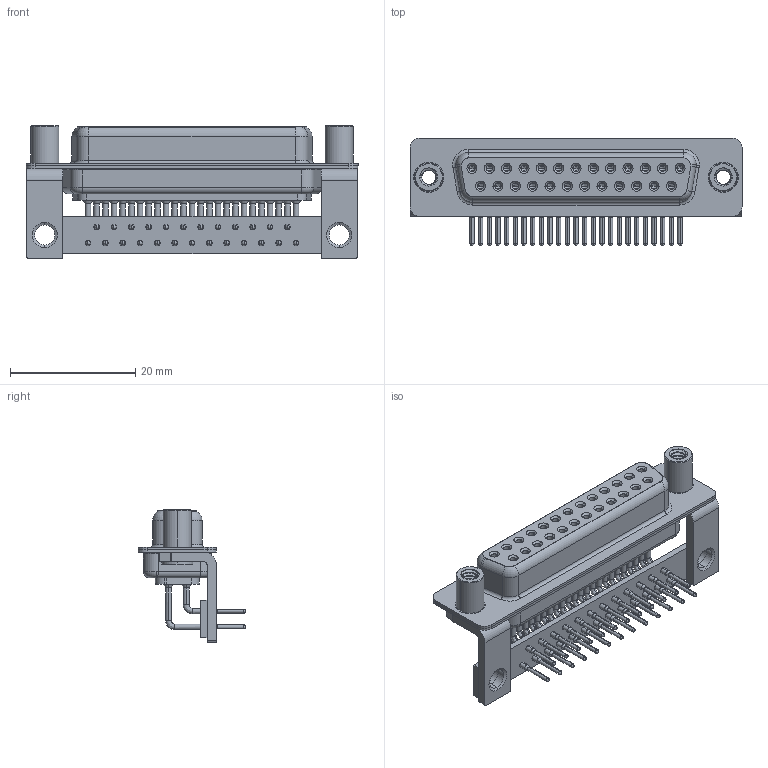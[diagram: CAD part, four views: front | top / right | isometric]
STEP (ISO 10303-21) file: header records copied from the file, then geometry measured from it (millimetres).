
FILE_DESCRIPTION (( 'STEP AP203' ), '1' );
FILE_NAME ('630-M25-640-GN6.STEP', '2018-09-26T03:07:29', ( '' ), ( '' ), 'SwSTEP 2.0', 'SolidWorks 2016', '' );
FILE_SCHEMA (( 'CONFIG_CONTROL_DESIGN' ));
Length unit declared in the file: millimetre
Products named in the file (9): 630M Shell Rear_25 Contacts; 630M Contact Row 1; 630M Contact Row 2; 630M Stabilizer Bracket; 630M 4-40 Threaded Standoff; 630M Stabilizer Board_25 Contacts; 630-M25-640-GN6; 630M Housing_25 Contacts; 630M Shell Front_25 Contacts
Assembly tree (33 placements, depth 2):
  630-M25-640-GN6
    630M Housing_25 Contacts
    630M Shell Front_25 Contacts
    630M Shell Rear_25 Contacts
    630M Contact Row 1  x13
    630M Contact Row 2  x12
    630M Stabilizer Bracket  x2
    630M 4-40 Threaded Standoff  x2
    630M Stabilizer Board_25 Contacts
Bounding box: 53.05 x 17.2 x 21.2 mm (x, y, z)
Volume: 4578.3 mm3; surface area: 11419.2 mm2
Topology: 33 solids, 33 shells, 1754 faces, 4480 edges, 2830 vertices
Faces by surface type: cylinder 826, plane 470, cone 289, bspline 106, torus 63
Entity records: 26098 total; most frequent: CARTESIAN_POINT 6001, DIRECTION 4219, ORIENTED_EDGE 3614, EDGE_CURVE 1807, AXIS2_PLACEMENT_3D 1758, VERTEX_POINT 1156, CIRCLE 977, EDGE_LOOP 967
